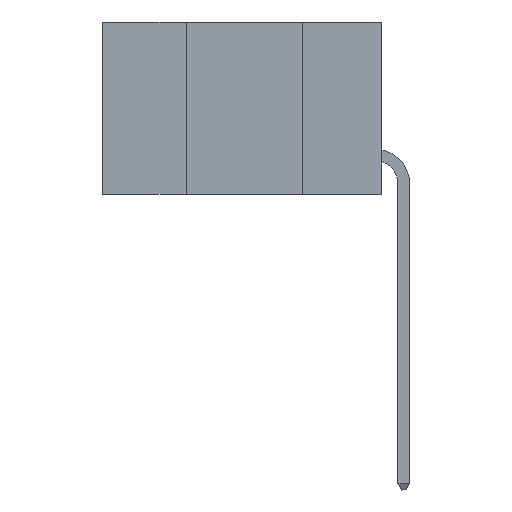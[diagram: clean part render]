
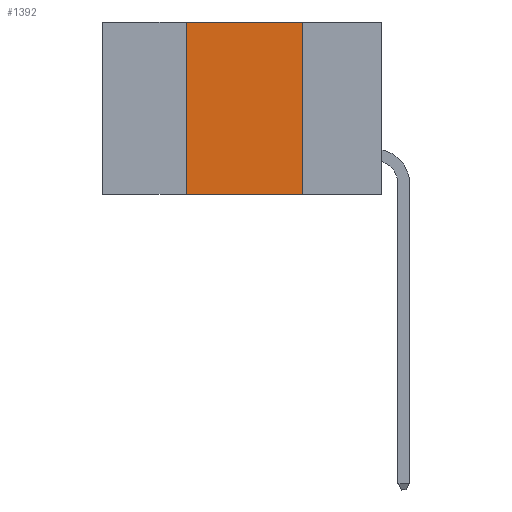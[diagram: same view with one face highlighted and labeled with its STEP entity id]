
A CAD part, left-side view. The second image highlights one B-rep face of the part: STEP entity #1392.
In plain terms, the highlighted planar face has unit normal (-1, 0, 0).
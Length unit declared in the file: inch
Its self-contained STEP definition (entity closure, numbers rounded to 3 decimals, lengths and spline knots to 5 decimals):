
#320 = EDGE_CURVE ( 'NONE', #3765, #7372, #849, .T. ) ;
#698 = EDGE_CURVE ( 'NONE', #9757, #3765, #5386, .T. ) ;
#849 = LINE ( 'NONE', #7197, #2227 ) ;
#904 = PLANE ( 'NONE',  #8833 ) ;
#1392 = ADVANCED_FACE ( 'NONE', ( #5489 ), #904, .F. ) ;
#1578 = CARTESIAN_POINT ( 'NONE',  ( 0., 0.42, 0. ) ) ;
#1802 = CARTESIAN_POINT ( 'NONE',  ( 0., 0.17, 0. ) ) ;
#2227 = VECTOR ( 'NONE', #8907, 39.37008 ) ;
#3140 = CARTESIAN_POINT ( 'NONE',  ( 0., 0.42, -0.37 ) ) ;
#3765 = VERTEX_POINT ( 'NONE', #1802 ) ;
#3884 = EDGE_LOOP ( 'NONE', ( #7177, #10266, #8126, #10554 ) ) ;
#4015 = CARTESIAN_POINT ( 'NONE',  ( 0., 0.17, -0.37 ) ) ;
#4120 = DIRECTION ( 'NONE',  ( 0., 0., -1. ) ) ;
#4175 = CARTESIAN_POINT ( 'NONE',  ( 0., 0.6, -0.37 ) ) ;
#4258 = VECTOR ( 'NONE', #6555, 39.37008 ) ;
#5062 = LINE ( 'NONE', #9997, #5878 ) ;
#5149 = EDGE_CURVE ( 'NONE', #11197, #9757, #5062, .T. ) ;
#5386 = LINE ( 'NONE', #8169, #9810 ) ;
#5489 = FACE_OUTER_BOUND ( 'NONE', #3884, .T. ) ;
#5878 = VECTOR ( 'NONE', #8227, 39.37008 ) ;
#6555 = DIRECTION ( 'NONE',  ( 0., -1., 0. ) ) ;
#7177 = ORIENTED_EDGE ( 'NONE', *, *, #320, .F. ) ;
#7197 = CARTESIAN_POINT ( 'NONE',  ( 0., 0.17, 0. ) ) ;
#7372 = VERTEX_POINT ( 'NONE', #4015 ) ;
#8126 = ORIENTED_EDGE ( 'NONE', *, *, #5149, .F. ) ;
#8169 = CARTESIAN_POINT ( 'NONE',  ( 0., 0.6, 0. ) ) ;
#8227 = DIRECTION ( 'NONE',  ( 0., 0., 1. ) ) ;
#8833 = AXIS2_PLACEMENT_3D ( 'NONE', #8862, #11236, #4120 ) ;
#8862 = CARTESIAN_POINT ( 'NONE',  ( 0., 0.6, 0. ) ) ;
#8907 = DIRECTION ( 'NONE',  ( 0., 0., -1. ) ) ;
#9757 = VERTEX_POINT ( 'NONE', #1578 ) ;
#9761 = EDGE_CURVE ( 'NONE', #11197, #7372, #11055, .T. ) ;
#9790 = DIRECTION ( 'NONE',  ( 0., -1., 0. ) ) ;
#9810 = VECTOR ( 'NONE', #9790, 39.37008 ) ;
#9997 = CARTESIAN_POINT ( 'NONE',  ( 0., 0.42, 0. ) ) ;
#10266 = ORIENTED_EDGE ( 'NONE', *, *, #698, .F. ) ;
#10554 = ORIENTED_EDGE ( 'NONE', *, *, #9761, .T. ) ;
#11055 = LINE ( 'NONE', #4175, #4258 ) ;
#11197 = VERTEX_POINT ( 'NONE', #3140 ) ;
#11236 = DIRECTION ( 'NONE',  ( 1., 0., 0. ) ) ;
